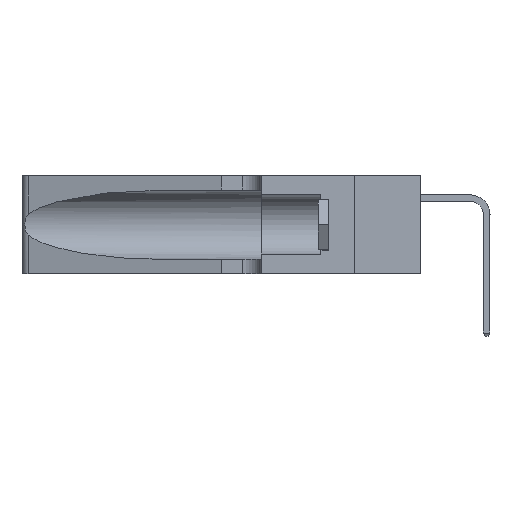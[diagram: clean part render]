
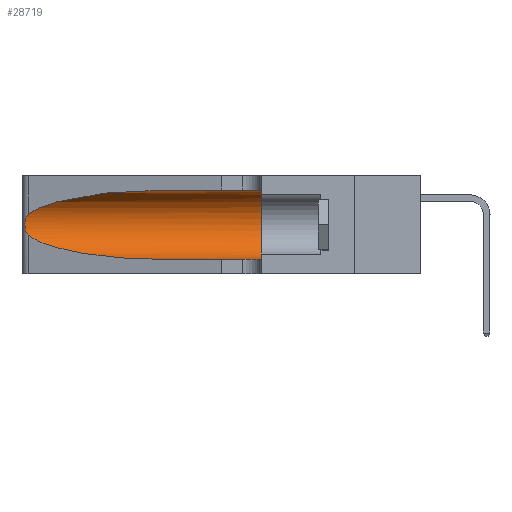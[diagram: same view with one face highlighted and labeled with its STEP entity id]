
A CAD part, left-side view. The second image highlights one B-rep face of the part: STEP entity #28719.
In plain terms, the highlighted cylindrical face has radius 3.308 mm (diameter 6.617 mm), a partial arc.
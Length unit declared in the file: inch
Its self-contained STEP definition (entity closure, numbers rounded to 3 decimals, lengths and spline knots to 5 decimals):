
#83 = CARTESIAN_POINT ( 'NONE',  ( 0.18966, 0.96281, 0.31525 ) ) ;
#1104 = CARTESIAN_POINT ( 'NONE',  ( 0.25487, 1.22718, 0.14631 ) ) ;
#1824 = CARTESIAN_POINT ( 'NONE',  ( 0.25639, 1.23186, 0.15144 ) ) ;
#2206 = ORIENTED_EDGE ( 'NONE', *, *, #23740, .T. ) ;
#3205 = VECTOR ( 'NONE', #41844, 39.37008 ) ;
#4835 = CARTESIAN_POINT ( 'NONE',  ( 0.1305, 0.72297, 0.05475 ) ) ;
#5556 = CARTESIAN_POINT ( 'NONE',  ( 0.25487, 1.22718, 0.14631 ) ) ;
#5791 = CARTESIAN_POINT ( 'NONE',  ( 0.1305, 0.35, 0.185 ) ) ;
#6063 = VECTOR ( 'NONE', #41743, 39.37008 ) ;
#6085 = EDGE_CURVE ( 'NONE', #33111, #30105, #25051, .T. ) ;
#6230 = VERTEX_POINT ( 'NONE', #42292 ) ;
#6234 = EDGE_CURVE ( 'NONE', #6230, #25217, #30686, .T. ) ;
#6714 = AXIS2_PLACEMENT_3D ( 'NONE', #26954, #16069, #8617 ) ;
#7210 = LINE ( 'NONE', #38094, #6063 ) ;
#7499 = CARTESIAN_POINT ( 'NONE',  ( 0.2373, 1.15595, 0.28018 ) ) ;
#8347 = CARTESIAN_POINT ( 'NONE',  ( 0.25487, 1.22718, 0.14631 ) ) ;
#8617 = DIRECTION ( 'NONE',  ( 0., 0., -1. ) ) ;
#9021 = CARTESIAN_POINT ( 'NONE',  ( 0.1305, 1.61858, 0.31525 ) ) ;
#9077 = CARTESIAN_POINT ( 'NONE',  ( 0.25639, 1.23184, 0.21858 ) ) ;
#9257 = EDGE_CURVE ( 'NONE', #46514, #6230, #32549, .T. ) ;
#9468 = DIRECTION ( 'NONE',  ( 0., 0., 1. ) ) ;
#12679 =( BOUNDED_CURVE ( )  B_SPLINE_CURVE ( 3, ( #25826, #83, #7499, #33223 ),
 .UNSPECIFIED., .F., .T. ) 
 B_SPLINE_CURVE_WITH_KNOTS ( ( 4, 4 ),
 ( 1.5708, 2.84003 ),
 .UNSPECIFIED. ) 
 CURVE ( )  GEOMETRIC_REPRESENTATION_ITEM ( )  RATIONAL_B_SPLINE_CURVE ( ( 1., 0.87, 0.87, 1. ) ) 
 REPRESENTATION_ITEM ( '' )  );
#12707 = VERTEX_POINT ( 'NONE', #26069 ) ;
#12810 = CARTESIAN_POINT ( 'NONE',  ( 0.25854, 1.2359, 0.20912 ) ) ;
#13731 = AXIS2_PLACEMENT_3D ( 'NONE', #5791, #31490, #9468 ) ;
#14440 = EDGE_CURVE ( 'NONE', #30105, #25217, #7210, .T. ) ;
#15352 = CARTESIAN_POINT ( 'NONE',  ( 0.1305, 0.72297, 0.31525 ) ) ;
#16069 = DIRECTION ( 'NONE',  ( 0., -1., 0. ) ) ;
#16357 = CARTESIAN_POINT ( 'NONE',  ( 0.25487, 1.22718, 0.22369 ) ) ;
#16515 = CARTESIAN_POINT ( 'NONE',  ( 0.26075, 1.23896, 0.19203 ) ) ;
#16731 = ORIENTED_EDGE ( 'NONE', *, *, #9257, .F. ) ;
#19562 = EDGE_CURVE ( 'NONE', #12707, #33111, #21204, .T. ) ;
#20181 = CARTESIAN_POINT ( 'NONE',  ( 0.26017, 1.23833, 0.17102 ) ) ;
#21204 = B_SPLINE_CURVE_WITH_KNOTS ( 'NONE', 3,
 ( #16357, #27385, #9077, #34779, #12810, #38402, #16515, #42042, #20181, #45698, #23855, #1824, #27551, #5556 ),
 .UNSPECIFIED., .F., .F.,
 ( 4, 2, 2, 2, 2, 2, 4 ),
 ( 0., 0.00027, 0.00053, 0.00107, 0.0016, 0.00187, 0.00214 ),
 .UNSPECIFIED. ) ;
#22429 = ORIENTED_EDGE ( 'NONE', *, *, #6085, .T. ) ;
#23740 = EDGE_CURVE ( 'NONE', #46514, #12707, #12679, .T. ) ;
#23855 = CARTESIAN_POINT ( 'NONE',  ( 0.25789, 1.23486, 0.15765 ) ) ;
#24468 = EDGE_LOOP ( 'NONE', ( #2206, #25845, #22429, #45856, #31689, #16731 ) ) ;
#25051 =( BOUNDED_CURVE ( )  B_SPLINE_CURVE ( 3, ( #1104, #37692, #30368, #4835 ),
 .UNSPECIFIED., .F., .T. ) 
 B_SPLINE_CURVE_WITH_KNOTS ( ( 4, 4 ),
 ( 3.44316, 4.71239 ),
 .UNSPECIFIED. ) 
 CURVE ( )  GEOMETRIC_REPRESENTATION_ITEM ( )  RATIONAL_B_SPLINE_CURVE ( ( 1., 0.87, 0.87, 1. ) ) 
 REPRESENTATION_ITEM ( '' )  );
#25217 = VERTEX_POINT ( 'NONE', #29598 ) ;
#25826 = CARTESIAN_POINT ( 'NONE',  ( 0.1305, 0.72297, 0.31525 ) ) ;
#25845 = ORIENTED_EDGE ( 'NONE', *, *, #19562, .T. ) ;
#26069 = CARTESIAN_POINT ( 'NONE',  ( 0.25487, 1.22718, 0.22369 ) ) ;
#26804 = CYLINDRICAL_SURFACE ( 'NONE', #6714, 0.13025 ) ;
#26954 = CARTESIAN_POINT ( 'NONE',  ( 0.1305, 1.61858, 0.185 ) ) ;
#27385 = CARTESIAN_POINT ( 'NONE',  ( 0.25555, 1.22994, 0.2215 ) ) ;
#27551 = CARTESIAN_POINT ( 'NONE',  ( 0.25555, 1.22993, 0.14849 ) ) ;
#28719 = ADVANCED_FACE ( 'NONE', ( #47313 ), #26804, .F. ) ;
#29598 = CARTESIAN_POINT ( 'NONE',  ( 0.1305, 0.35, 0.05475 ) ) ;
#30105 = VERTEX_POINT ( 'NONE', #31339 ) ;
#30368 = CARTESIAN_POINT ( 'NONE',  ( 0.18966, 0.96281, 0.05475 ) ) ;
#30686 = CIRCLE ( 'NONE', #13731, 0.13025 ) ;
#31339 = CARTESIAN_POINT ( 'NONE',  ( 0.1305, 0.72297, 0.05475 ) ) ;
#31490 = DIRECTION ( 'NONE',  ( 0., 1., 0. ) ) ;
#31689 = ORIENTED_EDGE ( 'NONE', *, *, #6234, .F. ) ;
#32549 = LINE ( 'NONE', #9021, #3205 ) ;
#33111 = VERTEX_POINT ( 'NONE', #8347 ) ;
#33223 = CARTESIAN_POINT ( 'NONE',  ( 0.25487, 1.22718, 0.22369 ) ) ;
#34779 = CARTESIAN_POINT ( 'NONE',  ( 0.25787, 1.23484, 0.2124 ) ) ;
#37692 = CARTESIAN_POINT ( 'NONE',  ( 0.2373, 1.15595, 0.08982 ) ) ;
#38094 = CARTESIAN_POINT ( 'NONE',  ( 0.1305, 1.61858, 0.05475 ) ) ;
#38402 = CARTESIAN_POINT ( 'NONE',  ( 0.26018, 1.23835, 0.19895 ) ) ;
#41743 = DIRECTION ( 'NONE',  ( 0., -1., 0. ) ) ;
#41844 = DIRECTION ( 'NONE',  ( 0., -1., 0. ) ) ;
#42042 = CARTESIAN_POINT ( 'NONE',  ( 0.26075, 1.23896, 0.178 ) ) ;
#42292 = CARTESIAN_POINT ( 'NONE',  ( 0.1305, 0.35, 0.31525 ) ) ;
#45698 = CARTESIAN_POINT ( 'NONE',  ( 0.25856, 1.23593, 0.16098 ) ) ;
#45856 = ORIENTED_EDGE ( 'NONE', *, *, #14440, .T. ) ;
#46514 = VERTEX_POINT ( 'NONE', #15352 ) ;
#47313 = FACE_OUTER_BOUND ( 'NONE', #24468, .T. ) ;
